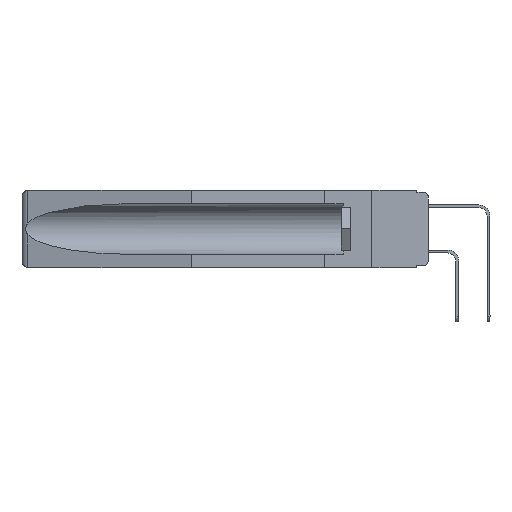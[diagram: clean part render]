
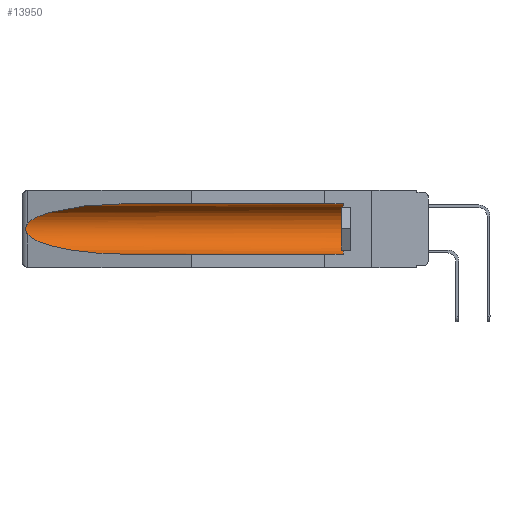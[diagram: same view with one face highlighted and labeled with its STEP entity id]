
A CAD part, left-side view. The second image highlights one B-rep face of the part: STEP entity #13950.
In plain terms, the highlighted cylindrical face has radius 2.857 mm (diameter 5.715 mm), a partial arc.
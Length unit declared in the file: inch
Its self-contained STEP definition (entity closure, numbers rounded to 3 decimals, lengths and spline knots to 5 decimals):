
#633 = CARTESIAN_POINT ( 'NONE',  ( 0.155, 1.07973, -0.059 ) ) ;
#714 = CARTESIAN_POINT ( 'NONE',  ( 0.155, 0.126, -0.059 ) ) ;
#1166 = CARTESIAN_POINT ( 'NONE',  ( 0.155, 1.07973, -0.059 ) ) ;
#1278 = CARTESIAN_POINT ( 'NONE',  ( 0.21114, 1.30732, -0.059 ) ) ;
#1690 = VERTEX_POINT ( 'NONE', #15153 ) ;
#1808 = CARTESIAN_POINT ( 'NONE',  ( 0.26537, 1.52718, -0.19328 ) ) ;
#2447 = CARTESIAN_POINT ( 'NONE',  ( 0.155, 1.07973, -0.284 ) ) ;
#2851 = DIRECTION ( 'NONE',  ( 0., 0., 1. ) ) ;
#3071 = CYLINDRICAL_SURFACE ( 'NONE', #12435, 0.1125 ) ;
#3337 = CARTESIAN_POINT ( 'NONE',  ( 0.2675, 1.53308, -0.16763 ) ) ;
#4087 = ORIENTED_EDGE ( 'NONE', *, *, #7704, .T. ) ;
#4126 =( BOUNDED_CURVE ( )  B_SPLINE_CURVE ( 3, ( #1166, #1278, #7992, #21785 ),
 .UNSPECIFIED., .F., .T. ) 
 B_SPLINE_CURVE_WITH_KNOTS ( ( 4, 4 ),
 ( 4.71239, 6.08839 ),
 .UNSPECIFIED. ) 
 CURVE ( )  GEOMETRIC_REPRESENTATION_ITEM ( )  RATIONAL_B_SPLINE_CURVE ( ( 1., 0.848, 0.848, 1. ) ) 
 REPRESENTATION_ITEM ( '' )  );
#5570 = CARTESIAN_POINT ( 'NONE',  ( 0.2673, 1.5327, -0.16383 ) ) ;
#5725 = EDGE_LOOP ( 'NONE', ( #7099, #8904, #6462, #21156, #4087, #13059 ) ) ;
#6141 = EDGE_CURVE ( 'NONE', #22045, #11346, #12551, .T. ) ;
#6449 = B_SPLINE_CURVE_WITH_KNOTS ( 'NONE', 3,
 ( #7238, #14064, #20919, #5570, #3337, #10158, #16986, #8490, #15291, #7820 ),
 .UNSPECIFIED., .F., .F.,
 ( 4, 2, 2, 2, 4 ),
 ( 0., 0.00029, 0.00058, 0.00087, 0.00117 ),
 .UNSPECIFIED. ) ;
#6462 = ORIENTED_EDGE ( 'NONE', *, *, #6141, .T. ) ;
#7099 = ORIENTED_EDGE ( 'NONE', *, *, #11850, .T. ) ;
#7238 = CARTESIAN_POINT ( 'NONE',  ( 0.26537, 1.52718, -0.14972 ) ) ;
#7289 = VECTOR ( 'NONE', #15117, 39.37008 ) ;
#7704 = EDGE_CURVE ( 'NONE', #1690, #16847, #19430, .T. ) ;
#7820 = CARTESIAN_POINT ( 'NONE',  ( 0.26537, 1.52718, -0.19328 ) ) ;
#7992 = CARTESIAN_POINT ( 'NONE',  ( 0.25451, 1.48313, -0.09465 ) ) ;
#8132 = DIRECTION ( 'NONE',  ( 0., 1., 0. ) ) ;
#8302 = LINE ( 'NONE', #18601, #7289 ) ;
#8490 = CARTESIAN_POINT ( 'NONE',  ( 0.26655, 1.53094, -0.18657 ) ) ;
#8635 = CARTESIAN_POINT ( 'NONE',  ( 0.155, 1.07973, -0.284 ) ) ;
#8904 = ORIENTED_EDGE ( 'NONE', *, *, #9864, .T. ) ;
#9864 = EDGE_CURVE ( 'NONE', #13820, #22045, #6449, .T. ) ;
#10029 = CARTESIAN_POINT ( 'NONE',  ( 0.155, -0.30754, -0.059 ) ) ;
#10158 = CARTESIAN_POINT ( 'NONE',  ( 0.2675, 1.53308, -0.17534 ) ) ;
#11346 = VERTEX_POINT ( 'NONE', #2447 ) ;
#11486 = EDGE_CURVE ( 'NONE', #16847, #19306, #11596, .T. ) ;
#11567 = FACE_OUTER_BOUND ( 'NONE', #5725, .T. ) ;
#11596 = LINE ( 'NONE', #10029, #21733 ) ;
#11850 = EDGE_CURVE ( 'NONE', #19306, #13820, #4126, .T. ) ;
#11914 = AXIS2_PLACEMENT_3D ( 'NONE', #13530, #21739, #14981 ) ;
#12435 = AXIS2_PLACEMENT_3D ( 'NONE', #14925, #21890, #2851 ) ;
#12551 =( BOUNDED_CURVE ( )  B_SPLINE_CURVE ( 3, ( #1808, #17473, #13654, #8635 ),
 .UNSPECIFIED., .F., .F. ) 
 B_SPLINE_CURVE_WITH_KNOTS ( ( 4, 4 ),
 ( 0.1948, 1.5708 ),
 .UNSPECIFIED. ) 
 CURVE ( )  GEOMETRIC_REPRESENTATION_ITEM ( )  RATIONAL_B_SPLINE_CURVE ( ( 1., 0.848, 0.848, 1. ) ) 
 REPRESENTATION_ITEM ( '' )  );
#13059 = ORIENTED_EDGE ( 'NONE', *, *, #11486, .T. ) ;
#13530 = CARTESIAN_POINT ( 'NONE',  ( 0.155, 0.126, -0.1715 ) ) ;
#13654 = CARTESIAN_POINT ( 'NONE',  ( 0.21114, 1.30732, -0.284 ) ) ;
#13820 = VERTEX_POINT ( 'NONE', #15945 ) ;
#13950 = ADVANCED_FACE ( 'NONE', ( #11567 ), #3071, .F. ) ;
#14064 = CARTESIAN_POINT ( 'NONE',  ( 0.26597, 1.52961, -0.15275 ) ) ;
#14925 = CARTESIAN_POINT ( 'NONE',  ( 0.155, -0.30754, -0.1715 ) ) ;
#14981 = DIRECTION ( 'NONE',  ( 0., 0., 1. ) ) ;
#15117 = DIRECTION ( 'NONE',  ( 0., 1., 0. ) ) ;
#15153 = CARTESIAN_POINT ( 'NONE',  ( 0.155, 0.126, -0.284 ) ) ;
#15291 = CARTESIAN_POINT ( 'NONE',  ( 0.26597, 1.5296, -0.19026 ) ) ;
#15945 = CARTESIAN_POINT ( 'NONE',  ( 0.26537, 1.52718, -0.14972 ) ) ;
#16847 = VERTEX_POINT ( 'NONE', #714 ) ;
#16981 = EDGE_CURVE ( 'NONE', #1690, #11346, #8302, .T. ) ;
#16986 = CARTESIAN_POINT ( 'NONE',  ( 0.2673, 1.53269, -0.17917 ) ) ;
#17473 = CARTESIAN_POINT ( 'NONE',  ( 0.25451, 1.48313, -0.24835 ) ) ;
#18601 = CARTESIAN_POINT ( 'NONE',  ( 0.155, -0.30754, -0.284 ) ) ;
#18766 = CARTESIAN_POINT ( 'NONE',  ( 0.26537, 1.52718, -0.19328 ) ) ;
#19306 = VERTEX_POINT ( 'NONE', #633 ) ;
#19430 = CIRCLE ( 'NONE', #11914, 0.1125 ) ;
#20919 = CARTESIAN_POINT ( 'NONE',  ( 0.26654, 1.53092, -0.15636 ) ) ;
#21156 = ORIENTED_EDGE ( 'NONE', *, *, #16981, .F. ) ;
#21733 = VECTOR ( 'NONE', #8132, 39.37008 ) ;
#21739 = DIRECTION ( 'NONE',  ( 0., -1., 0. ) ) ;
#21785 = CARTESIAN_POINT ( 'NONE',  ( 0.26537, 1.52718, -0.14972 ) ) ;
#21890 = DIRECTION ( 'NONE',  ( 0., 1., 0. ) ) ;
#22045 = VERTEX_POINT ( 'NONE', #18766 ) ;
